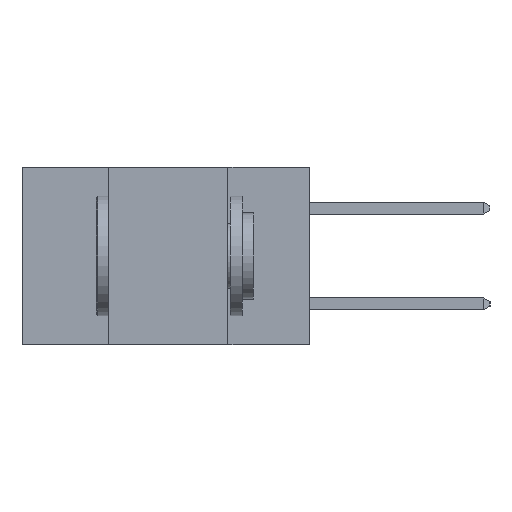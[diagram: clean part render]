
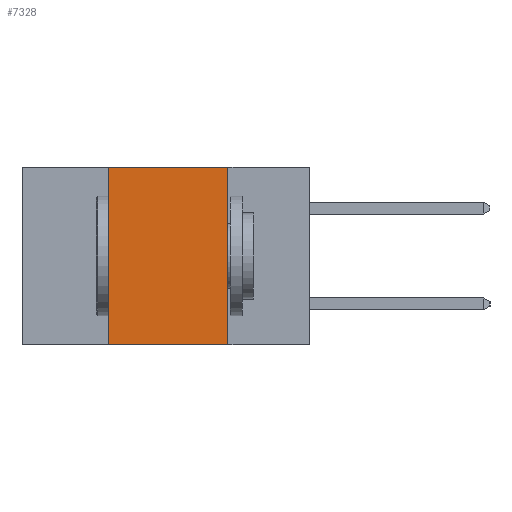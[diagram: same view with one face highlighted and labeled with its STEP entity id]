
A CAD part, left-side view. The second image highlights one B-rep face of the part: STEP entity #7328.
In plain terms, the highlighted planar face has unit normal (-1, 0, 0).
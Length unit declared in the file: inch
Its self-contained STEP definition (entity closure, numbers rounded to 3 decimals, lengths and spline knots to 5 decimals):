
#263 = EDGE_CURVE ( 'NONE', #13707, #2944, #5778, .T. ) ;
#504 = VECTOR ( 'NONE', #4624, 39.37008 ) ;
#508 = CARTESIAN_POINT ( 'NONE',  ( 0., 0.6, 0. ) ) ;
#2646 = PLANE ( 'NONE',  #3539 ) ;
#2944 = VERTEX_POINT ( 'NONE', #5312 ) ;
#3225 = EDGE_CURVE ( 'NONE', #10689, #8956, #11922, .T. ) ;
#3539 = AXIS2_PLACEMENT_3D ( 'NONE', #508, #12606, #8114 ) ;
#4624 = DIRECTION ( 'NONE',  ( 0., 0., 1. ) ) ;
#4647 = EDGE_CURVE ( 'NONE', #13707, #10689, #5370, .T. ) ;
#4825 = CARTESIAN_POINT ( 'NONE',  ( 0., 0.17, 0. ) ) ;
#5312 = CARTESIAN_POINT ( 'NONE',  ( 0., 0.17, -0.37 ) ) ;
#5370 = LINE ( 'NONE', #12212, #504 ) ;
#5778 = LINE ( 'NONE', #8949, #9392 ) ;
#5879 = CARTESIAN_POINT ( 'NONE',  ( 0., 0.42, 0. ) ) ;
#6096 = VECTOR ( 'NONE', #8967, 39.37008 ) ;
#7328 = ADVANCED_FACE ( 'NONE', ( #11891 ), #2646, .F. ) ;
#7958 = ORIENTED_EDGE ( 'NONE', *, *, #263, .T. ) ;
#8114 = DIRECTION ( 'NONE',  ( 0., 0., -1. ) ) ;
#8484 = ORIENTED_EDGE ( 'NONE', *, *, #12430, .F. ) ;
#8534 = ORIENTED_EDGE ( 'NONE', *, *, #4647, .F. ) ;
#8887 = CARTESIAN_POINT ( 'NONE',  ( 0., 0.6, 0. ) ) ;
#8949 = CARTESIAN_POINT ( 'NONE',  ( 0., 0.6, -0.37 ) ) ;
#8956 = VERTEX_POINT ( 'NONE', #11751 ) ;
#8967 = DIRECTION ( 'NONE',  ( 0., -1., 0. ) ) ;
#9177 = ORIENTED_EDGE ( 'NONE', *, *, #3225, .F. ) ;
#9392 = VECTOR ( 'NONE', #9969, 39.37008 ) ;
#9522 = VECTOR ( 'NONE', #11424, 39.37008 ) ;
#9865 = LINE ( 'NONE', #4825, #9522 ) ;
#9969 = DIRECTION ( 'NONE',  ( 0., -1., 0. ) ) ;
#10689 = VERTEX_POINT ( 'NONE', #5879 ) ;
#11424 = DIRECTION ( 'NONE',  ( 0., 0., -1. ) ) ;
#11751 = CARTESIAN_POINT ( 'NONE',  ( 0., 0.17, 0. ) ) ;
#11891 = FACE_OUTER_BOUND ( 'NONE', #13414, .T. ) ;
#11922 = LINE ( 'NONE', #8887, #6096 ) ;
#12212 = CARTESIAN_POINT ( 'NONE',  ( 0., 0.42, 0. ) ) ;
#12430 = EDGE_CURVE ( 'NONE', #8956, #2944, #9865, .T. ) ;
#12606 = DIRECTION ( 'NONE',  ( 1., 0., 0. ) ) ;
#13414 = EDGE_LOOP ( 'NONE', ( #8484, #9177, #8534, #7958 ) ) ;
#13553 = CARTESIAN_POINT ( 'NONE',  ( 0., 0.42, -0.37 ) ) ;
#13707 = VERTEX_POINT ( 'NONE', #13553 ) ;
